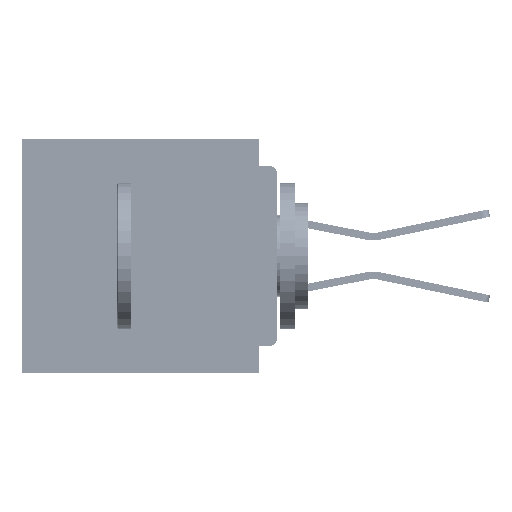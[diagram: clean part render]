
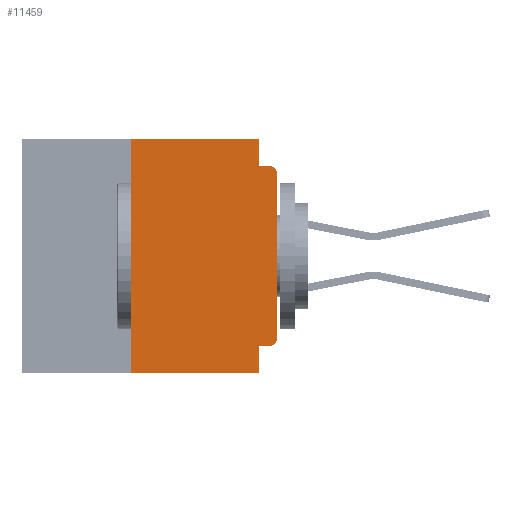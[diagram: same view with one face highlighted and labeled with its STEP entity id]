
A CAD part, left-side view. The second image highlights one B-rep face of the part: STEP entity #11459.
In plain terms, the highlighted planar face has unit normal (-1, 0, 0).
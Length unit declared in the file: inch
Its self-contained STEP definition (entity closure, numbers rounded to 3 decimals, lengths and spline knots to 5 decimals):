
#347 = VECTOR ( 'NONE', #33064, 39.37008 ) ;
#2009 = CARTESIAN_POINT ( 'NONE',  ( 0., 0.25, 0. ) ) ;
#2032 = LINE ( 'NONE', #11427, #347 ) ;
#2205 = DIRECTION ( 'NONE',  ( 0., -1., 0. ) ) ;
#3617 = VERTEX_POINT ( 'NONE', #49488 ) ;
#4194 = EDGE_CURVE ( 'NONE', #40174, #3617, #66435, .T. ) ;
#5756 = VERTEX_POINT ( 'NONE', #7589 ) ;
#5898 = FACE_OUTER_BOUND ( 'NONE', #24116, .T. ) ;
#6563 = VERTEX_POINT ( 'NONE', #62889 ) ;
#6720 = ORIENTED_EDGE ( 'NONE', *, *, #35925, .F. ) ;
#7589 = CARTESIAN_POINT ( 'NONE',  ( 0., 0.031, -0.355 ) ) ;
#7989 = CARTESIAN_POINT ( 'NONE',  ( 0., 0.437, 0. ) ) ;
#8271 = VERTEX_POINT ( 'NONE', #2009 ) ;
#9477 = EDGE_CURVE ( 'NONE', #6563, #30233, #62254, .T. ) ;
#9705 = EDGE_CURVE ( 'NONE', #58240, #48985, #33142, .T. ) ;
#10168 = LINE ( 'NONE', #30671, #65285 ) ;
#11427 = CARTESIAN_POINT ( 'NONE',  ( 0., 0.437, 0. ) ) ;
#11459 = ADVANCED_FACE ( 'NONE', ( #5898 ), #61541, .F. ) ;
#12728 = VECTOR ( 'NONE', #2205, 39.37008 ) ;
#12962 = DIRECTION ( 'NONE',  ( 0., 0., -1. ) ) ;
#14835 = CARTESIAN_POINT ( 'NONE',  ( 0., 0.015, -0.06 ) ) ;
#18579 = ORIENTED_EDGE ( 'NONE', *, *, #9477, .F. ) ;
#18887 = CARTESIAN_POINT ( 'NONE',  ( 0., 0.25, -0.4 ) ) ;
#20206 = DIRECTION ( 'NONE',  ( 0., 0., -1. ) ) ;
#20479 = EDGE_CURVE ( 'NONE', #37565, #8271, #50839, .T. ) ;
#21184 = LINE ( 'NONE', #52305, #33840 ) ;
#23606 = LINE ( 'NONE', #29025, #12728 ) ;
#23946 = VECTOR ( 'NONE', #56329, 39.37008 ) ;
#24116 = EDGE_LOOP ( 'NONE', ( #55872, #44211, #25460, #18579, #6720, #46963, #48679, #53844, #28623, #43454 ) ) ;
#25460 = ORIENTED_EDGE ( 'NONE', *, *, #69197, .F. ) ;
#25936 = DIRECTION ( 'NONE',  ( 0., 1., 0. ) ) ;
#26700 = CARTESIAN_POINT ( 'NONE',  ( 0., 0.25, -0.4 ) ) ;
#28514 = DIRECTION ( 'NONE',  ( 0., 0., -1. ) ) ;
#28569 = DIRECTION ( 'NONE',  ( -1., 0., 0. ) ) ;
#28586 = CARTESIAN_POINT ( 'NONE',  ( 0., 0.015, -0.34 ) ) ;
#28623 = ORIENTED_EDGE ( 'NONE', *, *, #53649, .F. ) ;
#29025 = CARTESIAN_POINT ( 'NONE',  ( 0., 0.437, -0.4 ) ) ;
#29625 = DIRECTION ( 'NONE',  ( 1., 0., 0. ) ) ;
#30233 = VERTEX_POINT ( 'NONE', #47743 ) ;
#30671 = CARTESIAN_POINT ( 'NONE',  ( 0., 0.031, -0.4 ) ) ;
#30989 = VERTEX_POINT ( 'NONE', #64265 ) ;
#33064 = DIRECTION ( 'NONE',  ( 0., -1., 0. ) ) ;
#33142 = CIRCLE ( 'NONE', #69126, 0.015 ) ;
#33840 = VECTOR ( 'NONE', #46930, 39.37008 ) ;
#35925 = EDGE_CURVE ( 'NONE', #8271, #6563, #2032, .T. ) ;
#36128 = DIRECTION ( 'NONE',  ( 0., 0., -1. ) ) ;
#37439 = VECTOR ( 'NONE', #12962, 39.37008 ) ;
#37565 = VERTEX_POINT ( 'NONE', #26700 ) ;
#37762 = CARTESIAN_POINT ( 'NONE',  ( 0., 0., -0.045 ) ) ;
#37823 = EDGE_CURVE ( 'NONE', #37565, #30989, #23606, .T. ) ;
#38017 = EDGE_CURVE ( 'NONE', #5756, #30989, #10168, .T. ) ;
#39438 = VECTOR ( 'NONE', #25936, 39.37008 ) ;
#40174 = VERTEX_POINT ( 'NONE', #65415 ) ;
#40508 = EDGE_CURVE ( 'NONE', #3617, #58240, #21184, .T. ) ;
#41347 = LINE ( 'NONE', #37762, #55500 ) ;
#41944 = CARTESIAN_POINT ( 'NONE',  ( 0., 0., -0.355 ) ) ;
#42853 = DIRECTION ( 'NONE',  ( 0., -1., 0. ) ) ;
#43183 = AXIS2_PLACEMENT_3D ( 'NONE', #28586, #28569, #28514 ) ;
#43454 = ORIENTED_EDGE ( 'NONE', *, *, #4194, .T. ) ;
#44211 = ORIENTED_EDGE ( 'NONE', *, *, #9705, .T. ) ;
#45130 = CARTESIAN_POINT ( 'NONE',  ( 0., 0.031, 0. ) ) ;
#46930 = DIRECTION ( 'NONE',  ( 0., 0., 1. ) ) ;
#46963 = ORIENTED_EDGE ( 'NONE', *, *, #20479, .F. ) ;
#47743 = CARTESIAN_POINT ( 'NONE',  ( 0., 0.031, -0.045 ) ) ;
#48679 = ORIENTED_EDGE ( 'NONE', *, *, #37823, .T. ) ;
#48985 = VERTEX_POINT ( 'NONE', #52432 ) ;
#49488 = CARTESIAN_POINT ( 'NONE',  ( 0., 0., -0.34 ) ) ;
#50839 = LINE ( 'NONE', #18887, #23946 ) ;
#52305 = CARTESIAN_POINT ( 'NONE',  ( 0., 0., 0. ) ) ;
#52344 = DIRECTION ( 'NONE',  ( -1., 0., 0. ) ) ;
#52432 = CARTESIAN_POINT ( 'NONE',  ( 0., 0.015, -0.045 ) ) ;
#53614 = LINE ( 'NONE', #41944, #39438 ) ;
#53649 = EDGE_CURVE ( 'NONE', #40174, #5756, #53614, .T. ) ;
#53844 = ORIENTED_EDGE ( 'NONE', *, *, #38017, .F. ) ;
#55500 = VECTOR ( 'NONE', #42853, 39.37008 ) ;
#55872 = ORIENTED_EDGE ( 'NONE', *, *, #40508, .T. ) ;
#56329 = DIRECTION ( 'NONE',  ( 0., 0., 1. ) ) ;
#57765 = AXIS2_PLACEMENT_3D ( 'NONE', #7989, #29625, #66848 ) ;
#58240 = VERTEX_POINT ( 'NONE', #68621 ) ;
#61541 = PLANE ( 'NONE',  #57765 ) ;
#62254 = LINE ( 'NONE', #45130, #37439 ) ;
#62889 = CARTESIAN_POINT ( 'NONE',  ( 0., 0.031, 0. ) ) ;
#64265 = CARTESIAN_POINT ( 'NONE',  ( 0., 0.031, -0.4 ) ) ;
#65285 = VECTOR ( 'NONE', #36128, 39.37008 ) ;
#65415 = CARTESIAN_POINT ( 'NONE',  ( 0., 0.015, -0.355 ) ) ;
#66435 = CIRCLE ( 'NONE', #43183, 0.015 ) ;
#66848 = DIRECTION ( 'NONE',  ( 0., 0., -1. ) ) ;
#68621 = CARTESIAN_POINT ( 'NONE',  ( 0., 0., -0.06 ) ) ;
#69126 = AXIS2_PLACEMENT_3D ( 'NONE', #14835, #52344, #20206 ) ;
#69197 = EDGE_CURVE ( 'NONE', #30233, #48985, #41347, .T. ) ;
